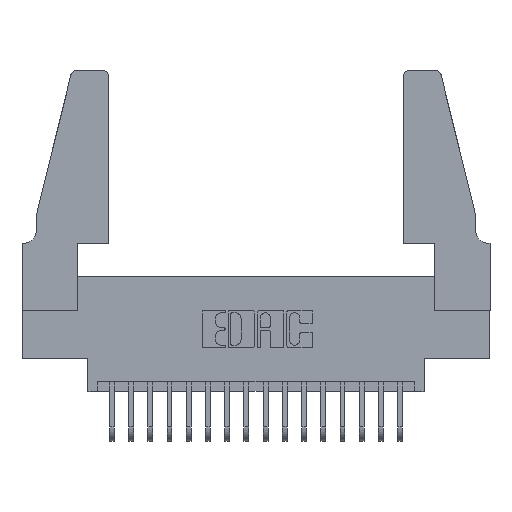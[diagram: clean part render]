
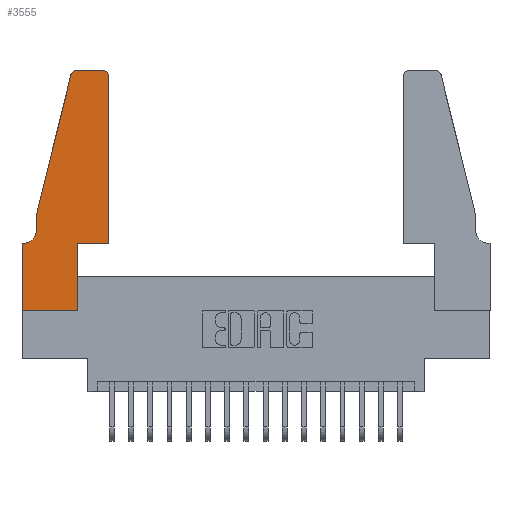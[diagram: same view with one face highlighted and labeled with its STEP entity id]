
A CAD part, top view. The second image highlights one B-rep face of the part: STEP entity #3555.
In plain terms, the highlighted planar face has unit normal (0, 0, 1).
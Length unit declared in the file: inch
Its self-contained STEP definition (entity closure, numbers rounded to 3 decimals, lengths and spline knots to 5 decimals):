
#105 = LINE ( 'NONE', #1535, #11644 ) ;
#121 = AXIS2_PLACEMENT_3D ( 'NONE', #11596, #6982, #17671 ) ;
#389 = FACE_OUTER_BOUND ( 'NONE', #13416, .T. ) ;
#1108 = AXIS2_PLACEMENT_3D ( 'NONE', #13210, #3966, #14728 ) ;
#1162 = VERTEX_POINT ( 'NONE', #15564 ) ;
#1284 = VERTEX_POINT ( 'NONE', #2034 ) ;
#1535 = CARTESIAN_POINT ( 'NONE',  ( 0.0755, 0.5, 0.37 ) ) ;
#1755 = AXIS2_PLACEMENT_3D ( 'NONE', #15680, #6518, #17203 ) ;
#2022 = VERTEX_POINT ( 'NONE', #4515 ) ;
#2034 = CARTESIAN_POINT ( 'NONE',  ( 0.2865, 0.35, 0.37 ) ) ;
#2246 = VERTEX_POINT ( 'NONE', #3212 ) ;
#2315 = CARTESIAN_POINT ( 'NONE',  ( 0., 0., 0.37 ) ) ;
#3212 = CARTESIAN_POINT ( 'NONE',  ( 0., 0.35, 0.37 ) ) ;
#3555 = ADVANCED_FACE ( 'NONE', ( #389 ), #16134, .T. ) ;
#3616 = DIRECTION ( 'NONE',  ( 0., 1., 0. ) ) ;
#3966 = DIRECTION ( 'NONE',  ( 0., 0., 1. ) ) ;
#4133 = ORIENTED_EDGE ( 'NONE', *, *, #13284, .T. ) ;
#4148 = CIRCLE ( 'NONE', #1755, 0.03 ) ;
#4515 = CARTESIAN_POINT ( 'NONE',  ( 0.2865, 0., 0.37 ) ) ;
#4734 = VECTOR ( 'NONE', #10117, 39.37008 ) ;
#4820 = ORIENTED_EDGE ( 'NONE', *, *, #5605, .T. ) ;
#4979 = CARTESIAN_POINT ( 'NONE',  ( 0.0055, 0.42, 0.37 ) ) ;
#5605 = EDGE_CURVE ( 'NONE', #13876, #6330, #12547, .T. ) ;
#5717 = CARTESIAN_POINT ( 'NONE',  ( 0.0755, 0.5, 0.37 ) ) ;
#6055 = ORIENTED_EDGE ( 'NONE', *, *, #14588, .T. ) ;
#6178 = ORIENTED_EDGE ( 'NONE', *, *, #10407, .T. ) ;
#6244 = LINE ( 'NONE', #16116, #13925 ) ;
#6266 = VERTEX_POINT ( 'NONE', #9648 ) ;
#6330 = VERTEX_POINT ( 'NONE', #18857 ) ;
#6518 = DIRECTION ( 'NONE',  ( 0., 0., 1. ) ) ;
#6543 = DIRECTION ( 'NONE',  ( -1., 0., 0. ) ) ;
#6760 = ORIENTED_EDGE ( 'NONE', *, *, #16608, .T. ) ;
#6892 = ORIENTED_EDGE ( 'NONE', *, *, #9697, .T. ) ;
#6964 = DIRECTION ( 'NONE',  ( 1., 0., 0. ) ) ;
#6982 = DIRECTION ( 'NONE',  ( 0., 0., 1. ) ) ;
#6983 = EDGE_CURVE ( 'NONE', #6330, #8605, #14171, .T. ) ;
#7064 = VERTEX_POINT ( 'NONE', #19416 ) ;
#7271 = VERTEX_POINT ( 'NONE', #19873 ) ;
#7303 = ORIENTED_EDGE ( 'NONE', *, *, #20008, .T. ) ;
#8116 = AXIS2_PLACEMENT_3D ( 'NONE', #4979, #15703, #6543 ) ;
#8442 = VECTOR ( 'NONE', #12174, 39.37008 ) ;
#8605 = VERTEX_POINT ( 'NONE', #20022 ) ;
#9138 = DIRECTION ( 'NONE',  ( -1., 0., 0. ) ) ;
#9139 = VECTOR ( 'NONE', #3616, 39.37008 ) ;
#9625 = EDGE_CURVE ( 'NONE', #6266, #7271, #16881, .T. ) ;
#9648 = CARTESIAN_POINT ( 'NONE',  ( 0.0755, 0.5, 0.37 ) ) ;
#9697 = EDGE_CURVE ( 'NONE', #1162, #2022, #15461, .T. ) ;
#9876 = VECTOR ( 'NONE', #18346, 39.37008 ) ;
#10117 = DIRECTION ( 'NONE',  ( 0., -1., 0. ) ) ;
#10353 = LINE ( 'NONE', #16820, #9876 ) ;
#10368 = CARTESIAN_POINT ( 'NONE',  ( 0.0055, 0.35, 0.37 ) ) ;
#10407 = EDGE_CURVE ( 'NONE', #8605, #6266, #105, .T. ) ;
#10489 = VERTEX_POINT ( 'NONE', #17141 ) ;
#10654 = CARTESIAN_POINT ( 'NONE',  ( 0.2605, 1.25, 0.37 ) ) ;
#11325 = ORIENTED_EDGE ( 'NONE', *, *, #19221, .T. ) ;
#11423 = VERTEX_POINT ( 'NONE', #10368 ) ;
#11456 = VECTOR ( 'NONE', #15120, 39.37008 ) ;
#11596 = CARTESIAN_POINT ( 'NONE',  ( 0., 0.35, 0.37 ) ) ;
#11644 = VECTOR ( 'NONE', #17010, 39.37008 ) ;
#11664 = ORIENTED_EDGE ( 'NONE', *, *, #9625, .T. ) ;
#12174 = DIRECTION ( 'NONE',  ( -1., 0., 0. ) ) ;
#12452 = EDGE_CURVE ( 'NONE', #1284, #10489, #6244, .T. ) ;
#12547 = LINE ( 'NONE', #10654, #8442 ) ;
#12879 = VECTOR ( 'NONE', #17967, 39.37008 ) ;
#13167 = VECTOR ( 'NONE', #9138, 39.37008 ) ;
#13210 = CARTESIAN_POINT ( 'NONE',  ( 0.284, 1.22, 0.37 ) ) ;
#13284 = EDGE_CURVE ( 'NONE', #2022, #1284, #10353, .T. ) ;
#13416 = EDGE_LOOP ( 'NONE', ( #4820, #17135, #6178, #11664, #18630, #6055, #7303, #6892, #4133, #15513, #11325, #6760 ) ) ;
#13628 = CARTESIAN_POINT ( 'NONE',  ( 0.4205, 1.25, 0.37 ) ) ;
#13876 = VERTEX_POINT ( 'NONE', #13628 ) ;
#13925 = VECTOR ( 'NONE', #6964, 39.37008 ) ;
#14171 = CIRCLE ( 'NONE', #1108, 0.03 ) ;
#14317 = CARTESIAN_POINT ( 'NONE',  ( 0.4505, 0.35, 0.37 ) ) ;
#14588 = EDGE_CURVE ( 'NONE', #11423, #2246, #17192, .T. ) ;
#14728 = DIRECTION ( 'NONE',  ( 1., 0., 0. ) ) ;
#15103 = CIRCLE ( 'NONE', #8116, 0.07 ) ;
#15120 = DIRECTION ( 'NONE',  ( 1., 0., 0. ) ) ;
#15461 = LINE ( 'NONE', #19613, #11456 ) ;
#15513 = ORIENTED_EDGE ( 'NONE', *, *, #12452, .T. ) ;
#15564 = CARTESIAN_POINT ( 'NONE',  ( 0., 0., 0.37 ) ) ;
#15680 = CARTESIAN_POINT ( 'NONE',  ( 0.4205, 1.22, 0.37 ) ) ;
#15703 = DIRECTION ( 'NONE',  ( 0., 0., -1. ) ) ;
#16116 = CARTESIAN_POINT ( 'NONE',  ( 0.4505, 0.35, 0.37 ) ) ;
#16134 = PLANE ( 'NONE',  #121 ) ;
#16269 = LINE ( 'NONE', #2315, #4734 ) ;
#16608 = EDGE_CURVE ( 'NONE', #7064, #13876, #4148, .T. ) ;
#16820 = CARTESIAN_POINT ( 'NONE',  ( 0.2865, 0.35, 0.37 ) ) ;
#16881 = LINE ( 'NONE', #5717, #12879 ) ;
#17010 = DIRECTION ( 'NONE',  ( -0.239, -0.971, 0. ) ) ;
#17135 = ORIENTED_EDGE ( 'NONE', *, *, #6983, .T. ) ;
#17141 = CARTESIAN_POINT ( 'NONE',  ( 0.4505, 0.35, 0.37 ) ) ;
#17192 = LINE ( 'NONE', #19757, #13167 ) ;
#17203 = DIRECTION ( 'NONE',  ( 1., 0., 0. ) ) ;
#17228 = LINE ( 'NONE', #14317, #9139 ) ;
#17671 = DIRECTION ( 'NONE',  ( 1., 0., 0. ) ) ;
#17967 = DIRECTION ( 'NONE',  ( 0., -1., 0. ) ) ;
#18346 = DIRECTION ( 'NONE',  ( 0., 1., 0. ) ) ;
#18630 = ORIENTED_EDGE ( 'NONE', *, *, #19143, .T. ) ;
#18857 = CARTESIAN_POINT ( 'NONE',  ( 0.284, 1.25, 0.37 ) ) ;
#19143 = EDGE_CURVE ( 'NONE', #7271, #11423, #15103, .T. ) ;
#19221 = EDGE_CURVE ( 'NONE', #10489, #7064, #17228, .T. ) ;
#19416 = CARTESIAN_POINT ( 'NONE',  ( 0.4505, 1.22, 0.37 ) ) ;
#19613 = CARTESIAN_POINT ( 'NONE',  ( 0., 0., 0.37 ) ) ;
#19757 = CARTESIAN_POINT ( 'NONE',  ( 0.0755, 0.35, 0.37 ) ) ;
#19873 = CARTESIAN_POINT ( 'NONE',  ( 0.0755, 0.42, 0.37 ) ) ;
#20008 = EDGE_CURVE ( 'NONE', #2246, #1162, #16269, .T. ) ;
#20022 = CARTESIAN_POINT ( 'NONE',  ( 0.25487, 1.22718, 0.37 ) ) ;
